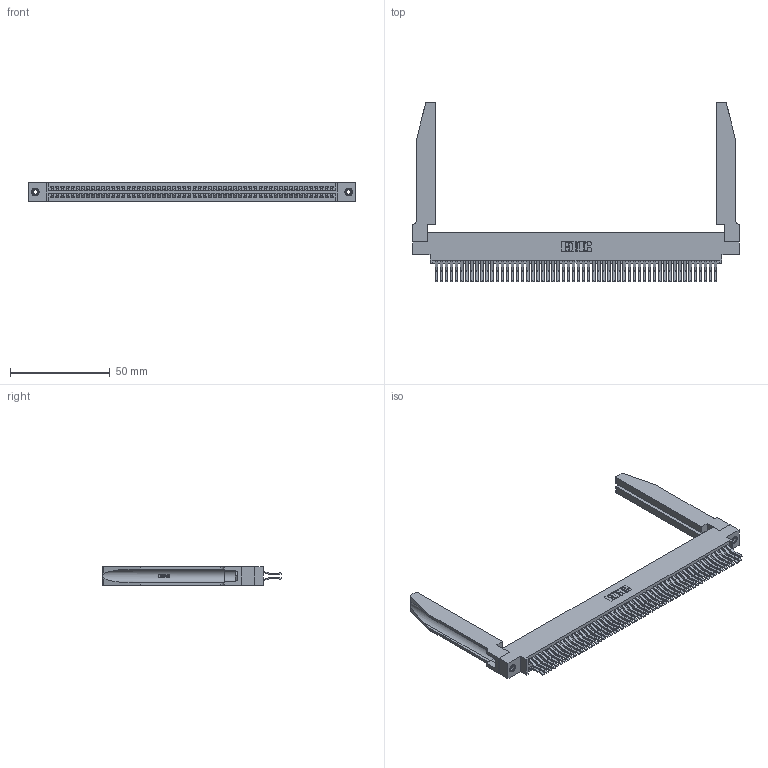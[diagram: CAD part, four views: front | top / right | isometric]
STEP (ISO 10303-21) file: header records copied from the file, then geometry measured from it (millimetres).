
FILE_DESCRIPTION (( 'STEP AP203' ), '1' );
FILE_NAME ('345-112-560-878.STEP', '2019-11-05T00:22:52', ( '' ), ( '' ), 'SwSTEP 2.0', 'SolidWorks 2016', '' );
FILE_SCHEMA (( 'CONFIG_CONTROL_DESIGN' ));
Length unit declared in the file: inch
Products named in the file (5): 345-292-001_560 Tail; 345-112-560-878; 345-220-078_345-220-078; 345 Part_0.170 Offset - 0.156 Dia-TH; 345-250-001_345-250-001-102
Assembly tree (117 placements, depth 2):
  345-112-560-878
    345 Part_0.170 Offset - 0.156 Dia-TH
    345-292-001_560 Tail  x112
    345-250-001_345-250-001-102  x2
    345-220-078_345-220-078  x2
Bounding box: 163.47 x 89.72 x 9.4 mm (x, y, z)
Volume: 24401.2 mm3; surface area: 33724.2 mm2
Topology: 117 solids, 117 shells, 6188 faces, 18321 edges, 12054 vertices
Faces by surface type: plane 3922, cylinder 2214, bspline 36, cone 12, torus 4
Entity records: 47014 total; most frequent: CARTESIAN_POINT 8787, ORIENTED_EDGE 7618, DIRECTION 6727, EDGE_CURVE 3809, VECTOR 3355, LINE 3355, VERTEX_POINT 2532, AXIS2_PLACEMENT_3D 1686
